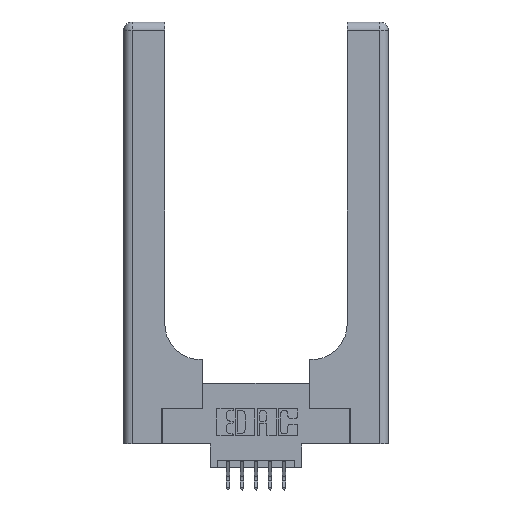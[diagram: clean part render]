
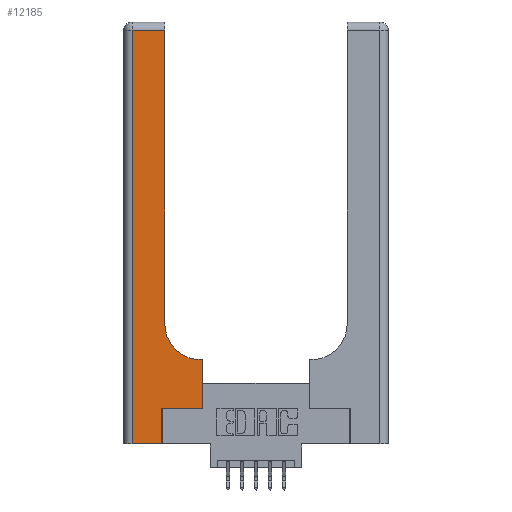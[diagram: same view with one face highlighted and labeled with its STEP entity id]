
A CAD part, top view. The second image highlights one B-rep face of the part: STEP entity #12185.
In plain terms, the highlighted planar face has unit normal (0, 0, 1).
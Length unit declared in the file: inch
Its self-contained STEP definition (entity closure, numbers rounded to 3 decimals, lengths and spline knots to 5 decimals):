
#498 = LINE ( 'NONE', #11301, #9386 ) ;
#557 = AXIS2_PLACEMENT_3D ( 'NONE', #1271, #2196, #7787 ) ;
#601 = FACE_OUTER_BOUND ( 'NONE', #8155, .T. ) ;
#698 = CARTESIAN_POINT ( 'NONE',  ( 0.5585, 0.25, 0.37 ) ) ;
#1107 = CARTESIAN_POINT ( 'NONE',  ( 0.5415, 0.6, 0.37 ) ) ;
#1172 = LINE ( 'NONE', #1598, #3971 ) ;
#1271 = CARTESIAN_POINT ( 'NONE',  ( 0.5415, 0.85, 0.37 ) ) ;
#1433 = EDGE_CURVE ( 'NONE', #7009, #4615, #12898, .T. ) ;
#1539 = CARTESIAN_POINT ( 'NONE',  ( 0.06, 2.94, 0.37 ) ) ;
#1598 = CARTESIAN_POINT ( 'NONE',  ( 0.2915, 3., 0.37 ) ) ;
#2196 = DIRECTION ( 'NONE',  ( 0., 0., -1. ) ) ;
#2432 = DIRECTION ( 'NONE',  ( 0., -1., 0. ) ) ;
#2471 = VERTEX_POINT ( 'NONE', #3141 ) ;
#2611 = CARTESIAN_POINT ( 'NONE',  ( 0.5585, 0.6, 0.37 ) ) ;
#3043 = VERTEX_POINT ( 'NONE', #7557 ) ;
#3141 = CARTESIAN_POINT ( 'NONE',  ( 0.269, 0., 0.37 ) ) ;
#3215 = VERTEX_POINT ( 'NONE', #8400 ) ;
#3246 = LINE ( 'NONE', #5900, #13903 ) ;
#3383 = CARTESIAN_POINT ( 'NONE',  ( 0.06, 0., 0.37 ) ) ;
#3401 = CARTESIAN_POINT ( 'NONE',  ( 0., 3., 0.37 ) ) ;
#3606 = VERTEX_POINT ( 'NONE', #4955 ) ;
#3971 = VECTOR ( 'NONE', #13715, 39.37008 ) ;
#3981 = DIRECTION ( 'NONE',  ( 0., 1., 0. ) ) ;
#4367 = ORIENTED_EDGE ( 'NONE', *, *, #9043, .T. ) ;
#4562 = ORIENTED_EDGE ( 'NONE', *, *, #6601, .T. ) ;
#4615 = VERTEX_POINT ( 'NONE', #1107 ) ;
#4845 = VERTEX_POINT ( 'NONE', #6311 ) ;
#4911 = AXIS2_PLACEMENT_3D ( 'NONE', #3401, #13412, #8949 ) ;
#4955 = CARTESIAN_POINT ( 'NONE',  ( 0.269, 0.25, 0.37 ) ) ;
#5615 = CARTESIAN_POINT ( 'NONE',  ( 0., 0., 0.37 ) ) ;
#5688 = EDGE_CURVE ( 'NONE', #3215, #10143, #5807, .T. ) ;
#5807 = LINE ( 'NONE', #10090, #11879 ) ;
#5900 = CARTESIAN_POINT ( 'NONE',  ( 0.269, 0., 0.37 ) ) ;
#6262 = CARTESIAN_POINT ( 'NONE',  ( 0.269, 0.25, 0.37 ) ) ;
#6311 = CARTESIAN_POINT ( 'NONE',  ( 0.5585, 0.25, 0.37 ) ) ;
#6601 = EDGE_CURVE ( 'NONE', #10143, #12837, #498, .T. ) ;
#6607 = ORIENTED_EDGE ( 'NONE', *, *, #14216, .T. ) ;
#6714 = DIRECTION ( 'NONE',  ( 1., 0., 0. ) ) ;
#6865 = LINE ( 'NONE', #6262, #10847 ) ;
#7009 = VERTEX_POINT ( 'NONE', #2611 ) ;
#7041 = EDGE_CURVE ( 'NONE', #4845, #7009, #13056, .T. ) ;
#7233 = ORIENTED_EDGE ( 'NONE', *, *, #9761, .T. ) ;
#7276 = EDGE_CURVE ( 'NONE', #12837, #2471, #7282, .T. ) ;
#7282 = LINE ( 'NONE', #5615, #11469 ) ;
#7283 = ORIENTED_EDGE ( 'NONE', *, *, #7041, .T. ) ;
#7557 = CARTESIAN_POINT ( 'NONE',  ( 0.2915, 0.85, 0.37 ) ) ;
#7698 = ORIENTED_EDGE ( 'NONE', *, *, #11547, .T. ) ;
#7787 = DIRECTION ( 'NONE',  ( 1., 0., 0. ) ) ;
#8155 = EDGE_LOOP ( 'NONE', ( #4367, #13338, #4562, #11429, #7698, #6607, #7283, #13747, #7233 ) ) ;
#8331 = DIRECTION ( 'NONE',  ( 1., 0., 0. ) ) ;
#8400 = CARTESIAN_POINT ( 'NONE',  ( 0.2915, 2.94, 0.37 ) ) ;
#8793 = PLANE ( 'NONE',  #4911 ) ;
#8935 = DIRECTION ( 'NONE',  ( -1., 0., 0. ) ) ;
#8949 = DIRECTION ( 'NONE',  ( -1., 0., 0. ) ) ;
#9043 = EDGE_CURVE ( 'NONE', #3043, #3215, #1172, .T. ) ;
#9386 = VECTOR ( 'NONE', #2432, 39.37008 ) ;
#9670 = CARTESIAN_POINT ( 'NONE',  ( 0.2915, 0.6, 0.37 ) ) ;
#9761 = EDGE_CURVE ( 'NONE', #4615, #3043, #12140, .T. ) ;
#9935 = VECTOR ( 'NONE', #14194, 39.37008 ) ;
#10090 = CARTESIAN_POINT ( 'NONE',  ( 0., 2.94, 0.37 ) ) ;
#10143 = VERTEX_POINT ( 'NONE', #1539 ) ;
#10847 = VECTOR ( 'NONE', #8331, 39.37008 ) ;
#11301 = CARTESIAN_POINT ( 'NONE',  ( 0.06, 3., 0.37 ) ) ;
#11429 = ORIENTED_EDGE ( 'NONE', *, *, #7276, .T. ) ;
#11469 = VECTOR ( 'NONE', #6714, 39.37008 ) ;
#11547 = EDGE_CURVE ( 'NONE', #2471, #3606, #3246, .T. ) ;
#11879 = VECTOR ( 'NONE', #8935, 39.37008 ) ;
#12140 = CIRCLE ( 'NONE', #557, 0.25 ) ;
#12185 = ADVANCED_FACE ( 'NONE', ( #601 ), #8793, .F. ) ;
#12696 = DIRECTION ( 'NONE',  ( 0., 1., 0. ) ) ;
#12837 = VERTEX_POINT ( 'NONE', #3383 ) ;
#12898 = LINE ( 'NONE', #9670, #9935 ) ;
#13056 = LINE ( 'NONE', #698, #14108 ) ;
#13338 = ORIENTED_EDGE ( 'NONE', *, *, #5688, .T. ) ;
#13412 = DIRECTION ( 'NONE',  ( 0., 0., -1. ) ) ;
#13715 = DIRECTION ( 'NONE',  ( 0., 1., 0. ) ) ;
#13747 = ORIENTED_EDGE ( 'NONE', *, *, #1433, .T. ) ;
#13903 = VECTOR ( 'NONE', #12696, 39.37008 ) ;
#14108 = VECTOR ( 'NONE', #3981, 39.37008 ) ;
#14194 = DIRECTION ( 'NONE',  ( -1., 0., 0. ) ) ;
#14216 = EDGE_CURVE ( 'NONE', #3606, #4845, #6865, .T. ) ;
